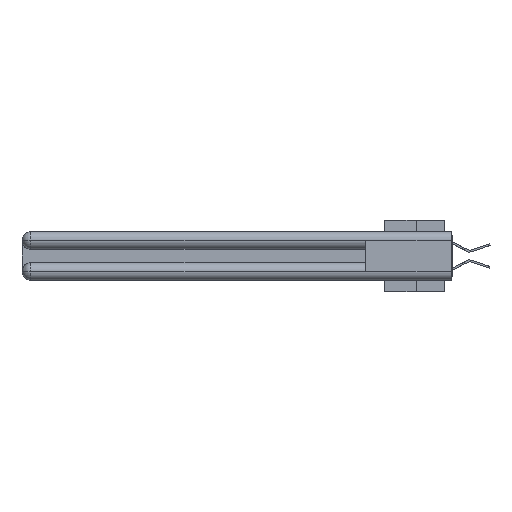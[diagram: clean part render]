
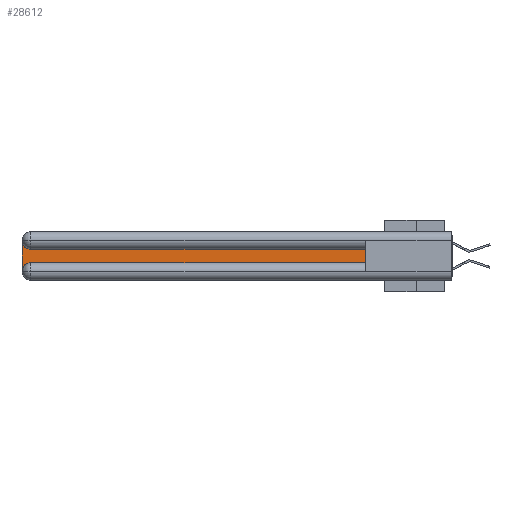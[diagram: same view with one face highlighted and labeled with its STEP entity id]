
A CAD part, left-side view. The second image highlights one B-rep face of the part: STEP entity #28612.
In plain terms, the highlighted planar face has unit normal (-1, 0, 0).
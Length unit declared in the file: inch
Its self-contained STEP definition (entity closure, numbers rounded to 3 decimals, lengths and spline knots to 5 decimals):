
#213 = ORIENTED_EDGE ( 'NONE', *, *, #22855, .T. ) ;
#1145 = PLANE ( 'NONE',  #24590 ) ;
#1163 = EDGE_CURVE ( 'NONE', #30848, #16335, #25494, .T. ) ;
#1380 = DIRECTION ( 'NONE',  ( 0., 0., -1. ) ) ;
#3050 = CARTESIAN_POINT ( 'NONE',  ( 0.075, 0.6, -0.2175 ) ) ;
#4004 = DIRECTION ( 'NONE',  ( 0., 0., -1. ) ) ;
#6026 = LINE ( 'NONE', #3050, #17863 ) ;
#7781 = CARTESIAN_POINT ( 'NONE',  ( 0.075, 0.6, -0.1225 ) ) ;
#8032 = EDGE_CURVE ( 'NONE', #16335, #17106, #23234, .T. ) ;
#8443 = AXIS2_PLACEMENT_3D ( 'NONE', #25474, #9462, #4004 ) ;
#9462 = DIRECTION ( 'NONE',  ( 1., 0., 0. ) ) ;
#10306 = VERTEX_POINT ( 'NONE', #19181 ) ;
#10371 = CARTESIAN_POINT ( 'NONE',  ( 0.075, 0.6, -0.1225 ) ) ;
#10675 = DIRECTION ( 'NONE',  ( 0., 0., -1. ) ) ;
#10993 = CIRCLE ( 'NONE', #29891, 0.06 ) ;
#11060 = DIRECTION ( 'NONE',  ( 0., 0., -1. ) ) ;
#12770 = VECTOR ( 'NONE', #34877, 39.37008 ) ;
#14507 = CARTESIAN_POINT ( 'NONE',  ( 0.075, 3., -0.2175 ) ) ;
#14781 = ORIENTED_EDGE ( 'NONE', *, *, #32041, .T. ) ;
#15009 = ORIENTED_EDGE ( 'NONE', *, *, #1163, .T. ) ;
#15809 = VERTEX_POINT ( 'NONE', #19744 ) ;
#16335 = VERTEX_POINT ( 'NONE', #27120 ) ;
#16385 = CARTESIAN_POINT ( 'NONE',  ( 0.075, 2.94, -0.2775 ) ) ;
#16864 = VECTOR ( 'NONE', #10675, 39.37008 ) ;
#17106 = VERTEX_POINT ( 'NONE', #33822 ) ;
#17619 = DIRECTION ( 'NONE',  ( 1., 0., 0. ) ) ;
#17863 = VECTOR ( 'NONE', #22011, 39.37008 ) ;
#18473 = VECTOR ( 'NONE', #32203, 39.37008 ) ;
#19181 = CARTESIAN_POINT ( 'NONE',  ( 0.075, 2.94, -0.2175 ) ) ;
#19744 = CARTESIAN_POINT ( 'NONE',  ( 0.075, 0.6, -0.2175 ) ) ;
#22011 = DIRECTION ( 'NONE',  ( 0., 0., 1. ) ) ;
#22153 = CARTESIAN_POINT ( 'NONE',  ( 0.075, 2.94, -0.1225 ) ) ;
#22855 = EDGE_CURVE ( 'NONE', #10306, #15809, #28487, .T. ) ;
#23234 = LINE ( 'NONE', #14507, #16864 ) ;
#23661 = VERTEX_POINT ( 'NONE', #7781 ) ;
#23955 = CARTESIAN_POINT ( 'NONE',  ( 0.075, 0.6, -0.2175 ) ) ;
#24590 = AXIS2_PLACEMENT_3D ( 'NONE', #28814, #17619, #1380 ) ;
#24628 = ORIENTED_EDGE ( 'NONE', *, *, #28459, .T. ) ;
#24731 = DIRECTION ( 'NONE',  ( 1., 0., 0. ) ) ;
#25474 = CARTESIAN_POINT ( 'NONE',  ( 0.075, 2.94, -0.0625 ) ) ;
#25494 = CIRCLE ( 'NONE', #8443, 0.06 ) ;
#25799 = EDGE_LOOP ( 'NONE', ( #29070, #15009, #32615, #14781, #213, #24628 ) ) ;
#26365 = FACE_OUTER_BOUND ( 'NONE', #25799, .T. ) ;
#27120 = CARTESIAN_POINT ( 'NONE',  ( 0.075, 3., -0.0625 ) ) ;
#28459 = EDGE_CURVE ( 'NONE', #15809, #23661, #6026, .T. ) ;
#28487 = LINE ( 'NONE', #23955, #12770 ) ;
#28612 = ADVANCED_FACE ( 'NONE', ( #26365 ), #1145, .F. ) ;
#28677 = LINE ( 'NONE', #10371, #18473 ) ;
#28814 = CARTESIAN_POINT ( 'NONE',  ( 0.075, 3., -0.1225 ) ) ;
#29070 = ORIENTED_EDGE ( 'NONE', *, *, #35179, .T. ) ;
#29891 = AXIS2_PLACEMENT_3D ( 'NONE', #16385, #24731, #11060 ) ;
#30848 = VERTEX_POINT ( 'NONE', #22153 ) ;
#32041 = EDGE_CURVE ( 'NONE', #17106, #10306, #10993, .T. ) ;
#32203 = DIRECTION ( 'NONE',  ( 0., 1., 0. ) ) ;
#32615 = ORIENTED_EDGE ( 'NONE', *, *, #8032, .T. ) ;
#33822 = CARTESIAN_POINT ( 'NONE',  ( 0.075, 3., -0.2775 ) ) ;
#34877 = DIRECTION ( 'NONE',  ( 0., -1., 0. ) ) ;
#35179 = EDGE_CURVE ( 'NONE', #23661, #30848, #28677, .T. ) ;
